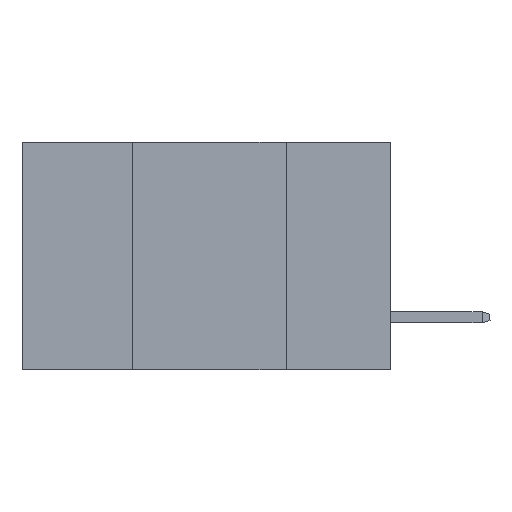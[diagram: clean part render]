
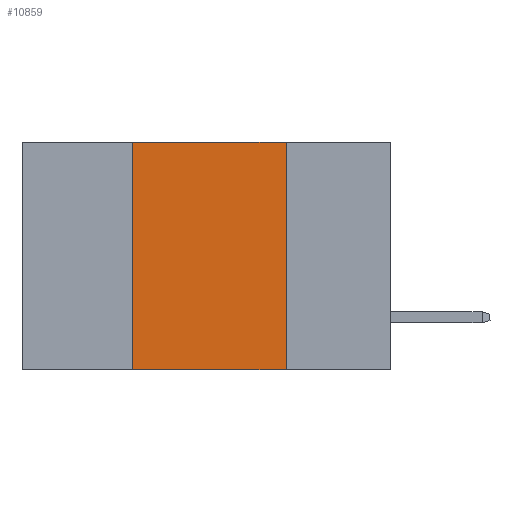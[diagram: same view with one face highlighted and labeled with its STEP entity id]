
A CAD part, left-side view. The second image highlights one B-rep face of the part: STEP entity #10859.
In plain terms, the highlighted planar face has unit normal (-1, 0, 0).
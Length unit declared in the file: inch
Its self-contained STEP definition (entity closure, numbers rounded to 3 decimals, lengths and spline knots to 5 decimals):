
#286 = DIRECTION ( 'NONE',  ( 0., -1., 0. ) ) ;
#688 = PLANE ( 'NONE',  #1748 ) ;
#815 = CARTESIAN_POINT ( 'NONE',  ( 0., 0.17, 0. ) ) ;
#935 = ORIENTED_EDGE ( 'NONE', *, *, #4367, .T. ) ;
#1123 = LINE ( 'NONE', #3544, #3043 ) ;
#1748 = AXIS2_PLACEMENT_3D ( 'NONE', #9806, #10393, #3649 ) ;
#2001 = VECTOR ( 'NONE', #7908, 39.37008 ) ;
#2254 = FACE_OUTER_BOUND ( 'NONE', #4738, .T. ) ;
#3043 = VECTOR ( 'NONE', #5206, 39.37008 ) ;
#3229 = LINE ( 'NONE', #815, #2001 ) ;
#3376 = CARTESIAN_POINT ( 'NONE',  ( 0., 0.42, -0.37 ) ) ;
#3544 = CARTESIAN_POINT ( 'NONE',  ( 0., 0.42, 0. ) ) ;
#3649 = DIRECTION ( 'NONE',  ( 0., 0., -1. ) ) ;
#3692 = CARTESIAN_POINT ( 'NONE',  ( 0., 0.17, 0. ) ) ;
#3764 = CARTESIAN_POINT ( 'NONE',  ( 0., 0.6, -0.37 ) ) ;
#3855 = VERTEX_POINT ( 'NONE', #11070 ) ;
#4276 = VERTEX_POINT ( 'NONE', #3692 ) ;
#4367 = EDGE_CURVE ( 'NONE', #8485, #3855, #6398, .T. ) ;
#4430 = VECTOR ( 'NONE', #9608, 39.37008 ) ;
#4738 = EDGE_LOOP ( 'NONE', ( #11351, #10535, #5135, #935 ) ) ;
#4793 = EDGE_CURVE ( 'NONE', #10231, #4276, #8610, .T. ) ;
#5135 = ORIENTED_EDGE ( 'NONE', *, *, #6282, .F. ) ;
#5206 = DIRECTION ( 'NONE',  ( 0., 0., 1. ) ) ;
#5309 = CARTESIAN_POINT ( 'NONE',  ( 0., 0.6, 0. ) ) ;
#5963 = VECTOR ( 'NONE', #286, 39.37008 ) ;
#6282 = EDGE_CURVE ( 'NONE', #8485, #10231, #1123, .T. ) ;
#6398 = LINE ( 'NONE', #3764, #5963 ) ;
#6863 = CARTESIAN_POINT ( 'NONE',  ( 0., 0.42, 0. ) ) ;
#7908 = DIRECTION ( 'NONE',  ( 0., 0., -1. ) ) ;
#8485 = VERTEX_POINT ( 'NONE', #3376 ) ;
#8610 = LINE ( 'NONE', #5309, #4430 ) ;
#9608 = DIRECTION ( 'NONE',  ( 0., -1., 0. ) ) ;
#9806 = CARTESIAN_POINT ( 'NONE',  ( 0., 0.6, 0. ) ) ;
#10073 = EDGE_CURVE ( 'NONE', #4276, #3855, #3229, .T. ) ;
#10231 = VERTEX_POINT ( 'NONE', #6863 ) ;
#10393 = DIRECTION ( 'NONE',  ( 1., 0., 0. ) ) ;
#10535 = ORIENTED_EDGE ( 'NONE', *, *, #4793, .F. ) ;
#10859 = ADVANCED_FACE ( 'NONE', ( #2254 ), #688, .F. ) ;
#11070 = CARTESIAN_POINT ( 'NONE',  ( 0., 0.17, -0.37 ) ) ;
#11351 = ORIENTED_EDGE ( 'NONE', *, *, #10073, .F. ) ;
